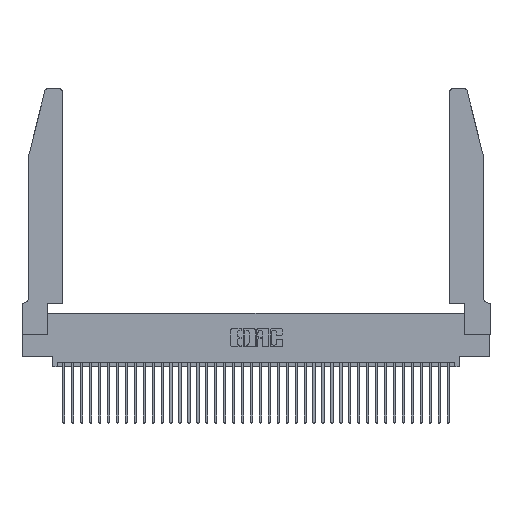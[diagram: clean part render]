
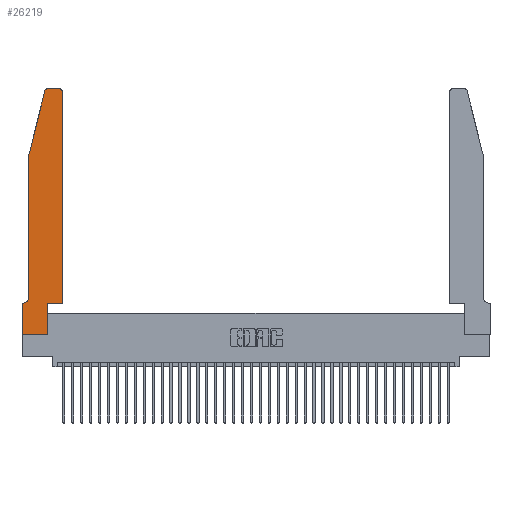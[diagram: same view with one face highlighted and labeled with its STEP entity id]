
A CAD part, top view. The second image highlights one B-rep face of the part: STEP entity #26219.
In plain terms, the highlighted planar face has unit normal (0, 0, 1).
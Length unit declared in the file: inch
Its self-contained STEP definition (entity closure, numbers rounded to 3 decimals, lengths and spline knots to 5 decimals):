
#51 = CARTESIAN_POINT ( 'NONE',  ( 0.25487, 2.72718, 0.37 ) ) ;
#802 = VERTEX_POINT ( 'NONE', #51 ) ;
#1120 = DIRECTION ( 'NONE',  ( 0., 1., 0. ) ) ;
#2848 = ORIENTED_EDGE ( 'NONE', *, *, #12725, .T. ) ;
#3579 = VERTEX_POINT ( 'NONE', #13211 ) ;
#3629 = AXIS2_PLACEMENT_3D ( 'NONE', #15795, #36618, #18842 ) ;
#3692 = CARTESIAN_POINT ( 'NONE',  ( 0.2605, 2.75, 0.37 ) ) ;
#4530 = CARTESIAN_POINT ( 'NONE',  ( 0.4505, 2.72, 0.37 ) ) ;
#4667 = AXIS2_PLACEMENT_3D ( 'NONE', #7929, #28993, #10999 ) ;
#5159 = ORIENTED_EDGE ( 'NONE', *, *, #34229, .T. ) ;
#5717 = ORIENTED_EDGE ( 'NONE', *, *, #37435, .T. ) ;
#5810 = VERTEX_POINT ( 'NONE', #32355 ) ;
#6408 = LINE ( 'NONE', #22527, #36467 ) ;
#6541 = CARTESIAN_POINT ( 'NONE',  ( 0., 0., 0.37 ) ) ;
#6797 = CARTESIAN_POINT ( 'NONE',  ( 0.0755, 2., 0.37 ) ) ;
#7445 = CARTESIAN_POINT ( 'NONE',  ( 0.2865, 0.35, 0.37 ) ) ;
#7882 = CARTESIAN_POINT ( 'NONE',  ( 0.4205, 2.72, 0.37 ) ) ;
#7929 = CARTESIAN_POINT ( 'NONE',  ( 0., 0.35, 0.37 ) ) ;
#8401 = FACE_OUTER_BOUND ( 'NONE', #13751, .T. ) ;
#8477 = CARTESIAN_POINT ( 'NONE',  ( 0.4505, 0.35, 0.37 ) ) ;
#8529 = VERTEX_POINT ( 'NONE', #13130 ) ;
#9895 = DIRECTION ( 'NONE',  ( -0.239, -0.971, 0. ) ) ;
#9896 = EDGE_CURVE ( 'NONE', #30663, #19302, #27706, .T. ) ;
#10256 = CIRCLE ( 'NONE', #22243, 0.03 ) ;
#10481 = DIRECTION ( 'NONE',  ( 1., 0., 0. ) ) ;
#10524 = ORIENTED_EDGE ( 'NONE', *, *, #9896, .T. ) ;
#10946 = DIRECTION ( 'NONE',  ( 1., 0., 0. ) ) ;
#10999 = DIRECTION ( 'NONE',  ( 1., 0., 0. ) ) ;
#11669 = VECTOR ( 'NONE', #1120, 39.37008 ) ;
#12038 = VECTOR ( 'NONE', #24630, 39.37008 ) ;
#12617 = ORIENTED_EDGE ( 'NONE', *, *, #35584, .T. ) ;
#12725 = EDGE_CURVE ( 'NONE', #19302, #36983, #22179, .T. ) ;
#13130 = CARTESIAN_POINT ( 'NONE',  ( 0., 0., 0.37 ) ) ;
#13211 = CARTESIAN_POINT ( 'NONE',  ( 0.0055, 0.35, 0.37 ) ) ;
#13751 = EDGE_LOOP ( 'NONE', ( #12617, #27779, #19413, #5159, #5717, #34582, #19802, #20329, #38437, #14367, #10524, #2848 ) ) ;
#13994 = LINE ( 'NONE', #6797, #21081 ) ;
#14253 = CARTESIAN_POINT ( 'NONE',  ( 0.2865, 0., 0.37 ) ) ;
#14367 = ORIENTED_EDGE ( 'NONE', *, *, #26064, .T. ) ;
#14452 = LINE ( 'NONE', #22854, #37295 ) ;
#15162 = VECTOR ( 'NONE', #36869, 39.37008 ) ;
#15282 = VECTOR ( 'NONE', #22392, 39.37008 ) ;
#15498 = EDGE_CURVE ( 'NONE', #3579, #17767, #35883, .T. ) ;
#15639 = DIRECTION ( 'NONE',  ( 1., 0., 0. ) ) ;
#15795 = CARTESIAN_POINT ( 'NONE',  ( 0.0055, 0.42, 0.37 ) ) ;
#15935 = CARTESIAN_POINT ( 'NONE',  ( 0.284, 2.72, 0.37 ) ) ;
#16224 = LINE ( 'NONE', #34176, #15282 ) ;
#16742 = VERTEX_POINT ( 'NONE', #23747 ) ;
#17767 = VERTEX_POINT ( 'NONE', #27172 ) ;
#17799 = VERTEX_POINT ( 'NONE', #36221 ) ;
#18842 = DIRECTION ( 'NONE',  ( -1., 0., 0. ) ) ;
#19000 = DIRECTION ( 'NONE',  ( 1., 0., 0. ) ) ;
#19302 = VERTEX_POINT ( 'NONE', #4530 ) ;
#19413 = ORIENTED_EDGE ( 'NONE', *, *, #32928, .T. ) ;
#19802 = ORIENTED_EDGE ( 'NONE', *, *, #33129, .T. ) ;
#20329 = ORIENTED_EDGE ( 'NONE', *, *, #30759, .T. ) ;
#21081 = VECTOR ( 'NONE', #9895, 39.37008 ) ;
#22179 = CIRCLE ( 'NONE', #36661, 0.03 ) ;
#22243 = AXIS2_PLACEMENT_3D ( 'NONE', #15935, #36781, #19000 ) ;
#22392 = DIRECTION ( 'NONE',  ( 0., -1., 0. ) ) ;
#22527 = CARTESIAN_POINT ( 'NONE',  ( 0.4505, 0.35, 0.37 ) ) ;
#22675 = CARTESIAN_POINT ( 'NONE',  ( 0.4205, 2.75, 0.37 ) ) ;
#22854 = CARTESIAN_POINT ( 'NONE',  ( 0., 0., 0.37 ) ) ;
#23173 = LINE ( 'NONE', #3692, #15162 ) ;
#23658 = VERTEX_POINT ( 'NONE', #14253 ) ;
#23712 = VERTEX_POINT ( 'NONE', #38346 ) ;
#23747 = CARTESIAN_POINT ( 'NONE',  ( 0.284, 2.75, 0.37 ) ) ;
#24008 = EDGE_CURVE ( 'NONE', #16742, #802, #10256, .T. ) ;
#24630 = DIRECTION ( 'NONE',  ( -1., 0., 0. ) ) ;
#25831 = DIRECTION ( 'NONE',  ( 0., -1., 0. ) ) ;
#25993 = VECTOR ( 'NONE', #15639, 39.37008 ) ;
#26064 = EDGE_CURVE ( 'NONE', #5810, #30663, #6408, .T. ) ;
#26219 = ADVANCED_FACE ( 'NONE', ( #8401 ), #37807, .T. ) ;
#27172 = CARTESIAN_POINT ( 'NONE',  ( 0., 0.35, 0.37 ) ) ;
#27231 = EDGE_CURVE ( 'NONE', #23658, #5810, #27660, .T. ) ;
#27660 = LINE ( 'NONE', #7445, #11669 ) ;
#27706 = LINE ( 'NONE', #8477, #34655 ) ;
#27779 = ORIENTED_EDGE ( 'NONE', *, *, #24008, .T. ) ;
#28950 = DIRECTION ( 'NONE',  ( 0., 0., 1. ) ) ;
#28993 = DIRECTION ( 'NONE',  ( 0., 0., 1. ) ) ;
#29611 = CARTESIAN_POINT ( 'NONE',  ( 0.4505, 0.35, 0.37 ) ) ;
#30663 = VERTEX_POINT ( 'NONE', #29611 ) ;
#30699 = CIRCLE ( 'NONE', #3629, 0.07 ) ;
#30759 = EDGE_CURVE ( 'NONE', #8529, #23658, #32902, .T. ) ;
#32355 = CARTESIAN_POINT ( 'NONE',  ( 0.2865, 0.35, 0.37 ) ) ;
#32496 = DIRECTION ( 'NONE',  ( 0., 1., 0. ) ) ;
#32902 = LINE ( 'NONE', #6541, #25993 ) ;
#32928 = EDGE_CURVE ( 'NONE', #802, #17799, #13994, .T. ) ;
#33129 = EDGE_CURVE ( 'NONE', #17767, #8529, #14452, .T. ) ;
#34176 = CARTESIAN_POINT ( 'NONE',  ( 0.0755, 2., 0.37 ) ) ;
#34229 = EDGE_CURVE ( 'NONE', #17799, #23712, #16224, .T. ) ;
#34582 = ORIENTED_EDGE ( 'NONE', *, *, #15498, .T. ) ;
#34655 = VECTOR ( 'NONE', #32496, 39.37008 ) ;
#35584 = EDGE_CURVE ( 'NONE', #36983, #16742, #23173, .T. ) ;
#35883 = LINE ( 'NONE', #36250, #12038 ) ;
#36221 = CARTESIAN_POINT ( 'NONE',  ( 0.0755, 2., 0.37 ) ) ;
#36250 = CARTESIAN_POINT ( 'NONE',  ( 0.0755, 0.35, 0.37 ) ) ;
#36467 = VECTOR ( 'NONE', #10481, 39.37008 ) ;
#36618 = DIRECTION ( 'NONE',  ( 0., 0., -1. ) ) ;
#36661 = AXIS2_PLACEMENT_3D ( 'NONE', #7882, #28950, #10946 ) ;
#36781 = DIRECTION ( 'NONE',  ( 0., 0., 1. ) ) ;
#36869 = DIRECTION ( 'NONE',  ( -1., 0., 0. ) ) ;
#36983 = VERTEX_POINT ( 'NONE', #22675 ) ;
#37295 = VECTOR ( 'NONE', #25831, 39.37008 ) ;
#37435 = EDGE_CURVE ( 'NONE', #23712, #3579, #30699, .T. ) ;
#37807 = PLANE ( 'NONE',  #4667 ) ;
#38346 = CARTESIAN_POINT ( 'NONE',  ( 0.0755, 0.42, 0.37 ) ) ;
#38437 = ORIENTED_EDGE ( 'NONE', *, *, #27231, .T. ) ;
